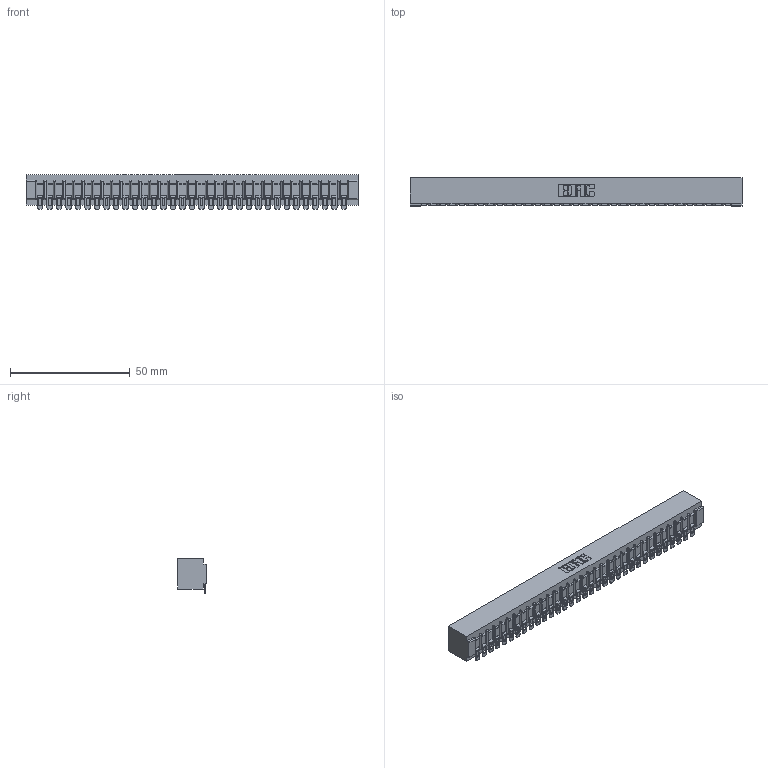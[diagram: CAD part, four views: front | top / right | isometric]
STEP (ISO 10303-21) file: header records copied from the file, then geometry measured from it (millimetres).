
FILE_DESCRIPTION (( 'STEP AP203' ), '1' );
FILE_NAME ('307-033-554-101.STEP', '2019-09-05T06:07:15', ( '' ), ( '' ), 'SwSTEP 2.0', 'SolidWorks 2016', '' );
FILE_SCHEMA (( 'CONFIG_CONTROL_DESIGN' ));
Length unit declared in the file: inch
Products named in the file (3): 307-290-002_554; 307-033-554-101; 307 Part_No Mounting Lugs
Assembly tree (34 placements, depth 2):
  307-033-554-101
    307 Part_No Mounting Lugs
    307-290-002_554  x33
Bounding box: 138.63 x 12.01 x 14.52 mm (x, y, z)
Volume: 15338 mm3; surface area: 19565.1 mm2
Topology: 34 solids, 34 shells, 2817 faces, 8648 edges, 5672 vertices
Faces by surface type: plane 1584, cylinder 1165, sphere 68
Entity records: 30087 total; most frequent: CARTESIAN_POINT 5074, ORIENTED_EDGE 5064, DIRECTION 4938, EDGE_CURVE 2532, LINE 1930, VECTOR 1930, VERTEX_POINT 1640, AXIS2_PLACEMENT_3D 1504
